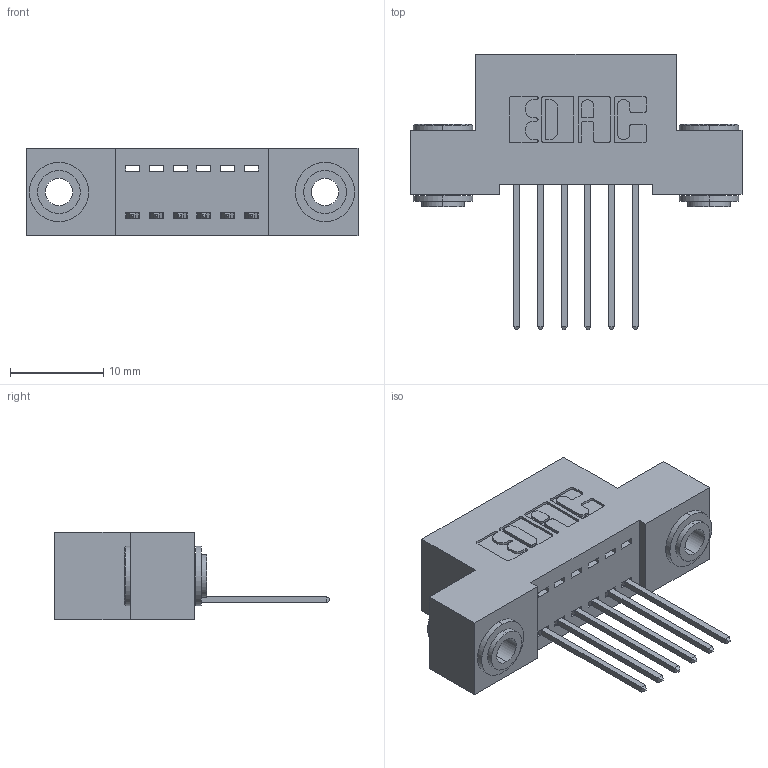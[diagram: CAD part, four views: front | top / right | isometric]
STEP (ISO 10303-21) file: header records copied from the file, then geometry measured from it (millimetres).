
FILE_DESCRIPTION (( 'STEP AP203' ), '1' );
FILE_NAME ('392-006-540-103.STEP', '2019-10-04T23:06:47', ( '' ), ( '' ), 'SwSTEP 2.0', 'SolidWorks 2016', '' );
FILE_SCHEMA (( 'CONFIG_CONTROL_DESIGN' ));
Length unit declared in the file: inch
Products named in the file (4): 392-006-540-103; 342 Part_.156 TH; 345-292-001_345-293-140; 342-250-002_345-250-002-102
Assembly tree (9 placements, depth 2):
  392-006-540-103
    342 Part_.156 TH
    345-292-001_345-293-140  x6
    342-250-002_345-250-002-102  x2
Bounding box: 35.56 x 29.47 x 9.4 mm (x, y, z)
Volume: 3016.2 mm3; surface area: 4039.4 mm2
Topology: 9 solids, 9 shells, 496 faces, 1431 edges, 942 vertices
Faces by surface type: plane 328, cylinder 160, cone 8
Entity records: 8860 total; most frequent: CARTESIAN_POINT 1511, ORIENTED_EDGE 1446, DIRECTION 1381, EDGE_CURVE 723, LINE 571, VECTOR 571, VERTEX_POINT 478, AXIS2_PLACEMENT_3D 405
